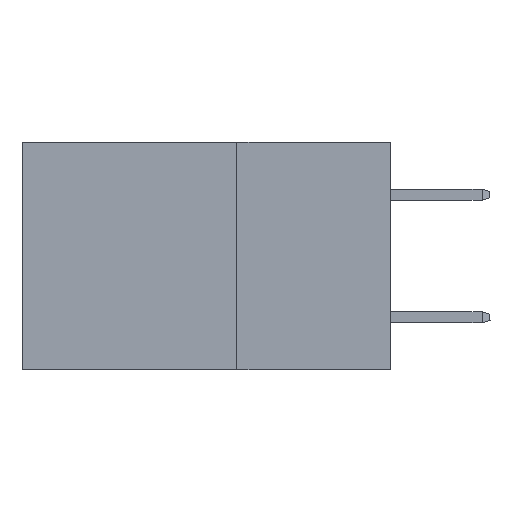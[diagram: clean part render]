
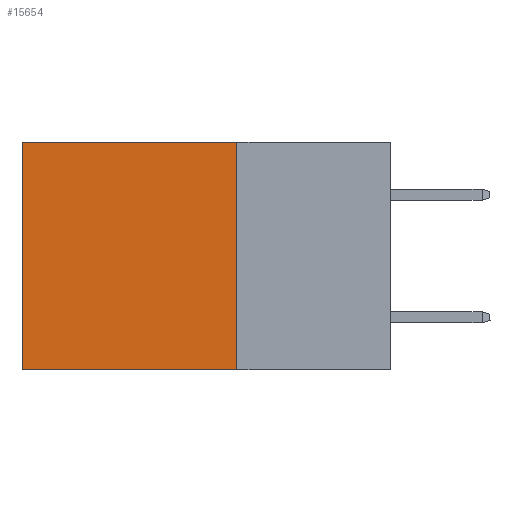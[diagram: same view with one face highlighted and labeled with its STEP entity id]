
A CAD part, left-side view. The second image highlights one B-rep face of the part: STEP entity #15654.
In plain terms, the highlighted planar face has unit normal (-1, 0, 0).
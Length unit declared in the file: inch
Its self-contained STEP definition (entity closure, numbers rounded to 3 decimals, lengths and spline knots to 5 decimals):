
#469 = CARTESIAN_POINT ( 'NONE',  ( 0.2875, 0.6, -0.37 ) ) ;
#971 = ORIENTED_EDGE ( 'NONE', *, *, #19003, .T. ) ;
#1515 = DIRECTION ( 'NONE',  ( 0., 0., -1. ) ) ;
#1784 = CARTESIAN_POINT ( 'NONE',  ( 0.2875, 0.25, 0. ) ) ;
#2958 = PLANE ( 'NONE',  #6517 ) ;
#4038 = LINE ( 'NONE', #1784, #10142 ) ;
#4348 = DIRECTION ( 'NONE',  ( 0., 0., -1. ) ) ;
#4670 = DIRECTION ( 'NONE',  ( 0., 1., 0. ) ) ;
#4962 = VECTOR ( 'NONE', #19148, 39.37008 ) ;
#5274 = VERTEX_POINT ( 'NONE', #469 ) ;
#6416 = VECTOR ( 'NONE', #4670, 39.37008 ) ;
#6517 = AXIS2_PLACEMENT_3D ( 'NONE', #27004, #29994, #11524 ) ;
#7080 = CARTESIAN_POINT ( 'NONE',  ( 0.2875, 0.25, -0.37 ) ) ;
#8169 = ORIENTED_EDGE ( 'NONE', *, *, #9097, .T. ) ;
#9021 = CARTESIAN_POINT ( 'NONE',  ( 0.2875, 0.6, 0. ) ) ;
#9097 = EDGE_CURVE ( 'NONE', #10578, #29779, #12072, .T. ) ;
#10142 = VECTOR ( 'NONE', #1515, 39.37008 ) ;
#10578 = VERTEX_POINT ( 'NONE', #28798 ) ;
#11524 = DIRECTION ( 'NONE',  ( 0., 0., -1. ) ) ;
#12072 = LINE ( 'NONE', #22664, #6416 ) ;
#12934 = LINE ( 'NONE', #7080, #4962 ) ;
#13399 = CARTESIAN_POINT ( 'NONE',  ( 0.2875, 0.6, 0. ) ) ;
#15654 = ADVANCED_FACE ( 'NONE', ( #21324 ), #2958, .F. ) ;
#16513 = EDGE_CURVE ( 'NONE', #28062, #5274, #12934, .T. ) ;
#18305 = VECTOR ( 'NONE', #4348, 39.37008 ) ;
#19003 = EDGE_CURVE ( 'NONE', #29779, #5274, #26327, .T. ) ;
#19148 = DIRECTION ( 'NONE',  ( 0., 1., 0. ) ) ;
#21324 = FACE_OUTER_BOUND ( 'NONE', #37021, .T. ) ;
#22664 = CARTESIAN_POINT ( 'NONE',  ( 0.2875, 0.25, 0. ) ) ;
#26327 = LINE ( 'NONE', #9021, #18305 ) ;
#27004 = CARTESIAN_POINT ( 'NONE',  ( 0.2875, 0.25, 0. ) ) ;
#28062 = VERTEX_POINT ( 'NONE', #32054 ) ;
#28798 = CARTESIAN_POINT ( 'NONE',  ( 0.2875, 0.25, 0. ) ) ;
#29779 = VERTEX_POINT ( 'NONE', #13399 ) ;
#29994 = DIRECTION ( 'NONE',  ( 1., 0., 0. ) ) ;
#32054 = CARTESIAN_POINT ( 'NONE',  ( 0.2875, 0.25, -0.37 ) ) ;
#33221 = ORIENTED_EDGE ( 'NONE', *, *, #34244, .F. ) ;
#34244 = EDGE_CURVE ( 'NONE', #10578, #28062, #4038, .T. ) ;
#37021 = EDGE_LOOP ( 'NONE', ( #971, #38101, #33221, #8169 ) ) ;
#38101 = ORIENTED_EDGE ( 'NONE', *, *, #16513, .F. ) ;
